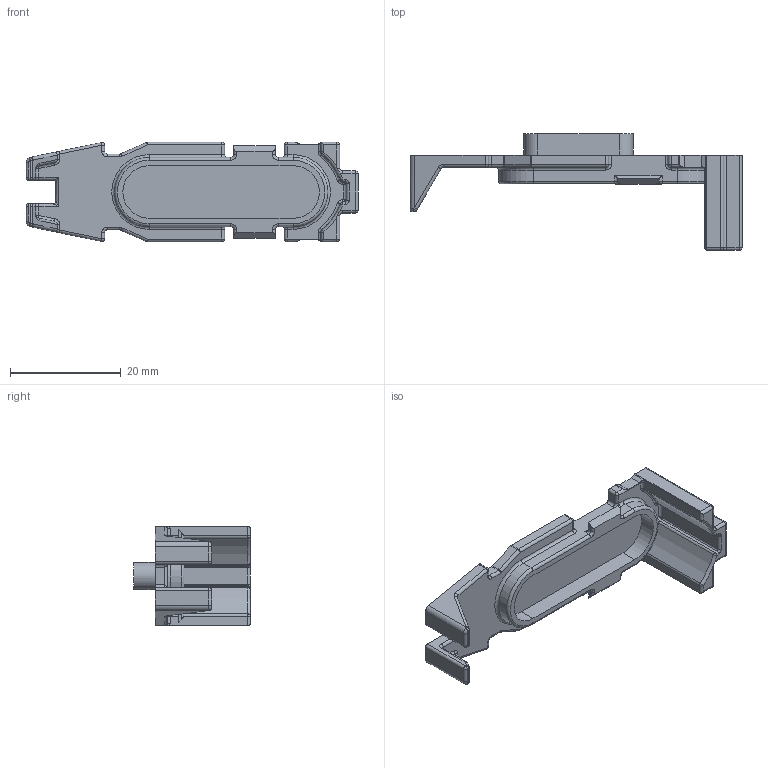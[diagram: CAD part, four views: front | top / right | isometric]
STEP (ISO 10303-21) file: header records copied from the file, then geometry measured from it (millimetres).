
FILE_DESCRIPTION (( 'STEP AP214' ), '1' );
FILE_NAME ('Base_Plate_Retainer.STEP', '2022-09-24T15:51:39', ( '' ), ( '' ), 'SwSTEP 2.0', 'SolidWorks 2021', '' );
FILE_SCHEMA (( 'AUTOMOTIVE_DESIGN' ));
Length unit declared in the file: millimetre
Products named in the file (1): Base_Plate_Retainer
Bounding box: 59.98 x 21.1 x 18 mm (x, y, z)
Volume: 3599 mm3; surface area: 3837.6 mm2
Topology: 1 solids, 1 shells, 273 faces, 669 edges, 373 vertices
Faces by surface type: cylinder 122, plane 76, torus 30, sphere 27, bspline 18
Entity records: 8037 total; most frequent: CARTESIAN_POINT 1869, DIRECTION 1334, ORIENTED_EDGE 1284, EDGE_CURVE 642, AXIS2_PLACEMENT_3D 509, VERTEX_POINT 373, LINE 316, VECTOR 316
